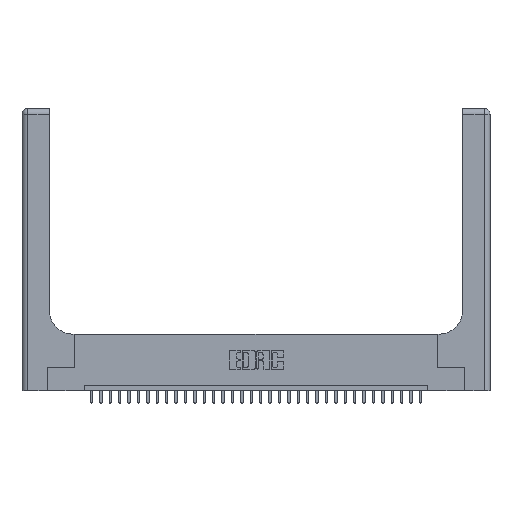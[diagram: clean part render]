
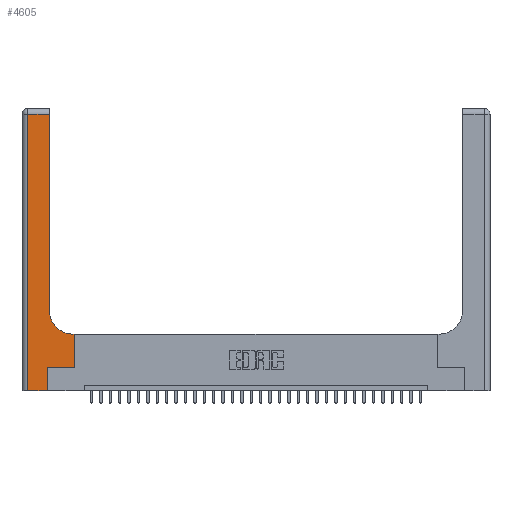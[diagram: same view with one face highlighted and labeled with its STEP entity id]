
A CAD part, top view. The second image highlights one B-rep face of the part: STEP entity #4605.
In plain terms, the highlighted planar face has unit normal (0, 0, 1).
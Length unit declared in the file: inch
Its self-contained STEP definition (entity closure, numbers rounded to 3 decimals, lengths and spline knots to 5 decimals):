
#498 = VERTEX_POINT ( 'NONE', #14320 ) ;
#702 = EDGE_CURVE ( 'NONE', #2515, #7853, #27507, .T. ) ;
#798 = DIRECTION ( 'NONE',  ( 1., 0., 0. ) ) ;
#1124 = CARTESIAN_POINT ( 'NONE',  ( 0.269, 0., 0.37 ) ) ;
#1391 = LINE ( 'NONE', #16752, #14208 ) ;
#1952 = VECTOR ( 'NONE', #13295, 39.37008 ) ;
#2410 = CARTESIAN_POINT ( 'NONE',  ( 0.5585, 0.25, 0.37 ) ) ;
#2515 = VERTEX_POINT ( 'NONE', #7560 ) ;
#3323 = CIRCLE ( 'NONE', #4582, 0.25 ) ;
#4096 = FACE_OUTER_BOUND ( 'NONE', #16424, .T. ) ;
#4129 = AXIS2_PLACEMENT_3D ( 'NONE', #18229, #7940, #10505 ) ;
#4148 = CARTESIAN_POINT ( 'NONE',  ( 0.269, 0.25, 0.37 ) ) ;
#4215 = LINE ( 'NONE', #9940, #5830 ) ;
#4252 = ORIENTED_EDGE ( 'NONE', *, *, #15939, .T. ) ;
#4377 = CARTESIAN_POINT ( 'NONE',  ( 0.269, 0., 0.37 ) ) ;
#4383 = CARTESIAN_POINT ( 'NONE',  ( 0.2915, 0.85, 0.37 ) ) ;
#4582 = AXIS2_PLACEMENT_3D ( 'NONE', #7587, #17984, #17672 ) ;
#4605 = ADVANCED_FACE ( 'NONE', ( #4096 ), #30809, .F. ) ;
#4661 = CARTESIAN_POINT ( 'NONE',  ( 0.5585, 0.25, 0.37 ) ) ;
#5014 = DIRECTION ( 'NONE',  ( 0., 1., 0. ) ) ;
#5274 = ORIENTED_EDGE ( 'NONE', *, *, #17654, .T. ) ;
#5356 = VECTOR ( 'NONE', #23576, 39.37008 ) ;
#5830 = VECTOR ( 'NONE', #15091, 39.37008 ) ;
#7560 = CARTESIAN_POINT ( 'NONE',  ( 0.06, 0., 0.37 ) ) ;
#7587 = CARTESIAN_POINT ( 'NONE',  ( 0.5415, 0.85, 0.37 ) ) ;
#7853 = VERTEX_POINT ( 'NONE', #1124 ) ;
#7940 = DIRECTION ( 'NONE',  ( 0., 0., -1. ) ) ;
#8458 = EDGE_CURVE ( 'NONE', #22135, #18496, #20179, .T. ) ;
#9336 = EDGE_CURVE ( 'NONE', #12132, #498, #11355, .T. ) ;
#9940 = CARTESIAN_POINT ( 'NONE',  ( 0.2915, 0.6, 0.37 ) ) ;
#10505 = DIRECTION ( 'NONE',  ( -1., 0., 0. ) ) ;
#10532 = VERTEX_POINT ( 'NONE', #10680 ) ;
#10680 = CARTESIAN_POINT ( 'NONE',  ( 0.06, 2.94, 0.37 ) ) ;
#11167 = EDGE_CURVE ( 'NONE', #7853, #28738, #30779, .T. ) ;
#11355 = LINE ( 'NONE', #13648, #5356 ) ;
#11925 = DIRECTION ( 'NONE',  ( 0., -1., 0. ) ) ;
#12132 = VERTEX_POINT ( 'NONE', #4383 ) ;
#12150 = DIRECTION ( 'NONE',  ( -1., 0., 0. ) ) ;
#12954 = CARTESIAN_POINT ( 'NONE',  ( 0., 0., 0.37 ) ) ;
#13295 = DIRECTION ( 'NONE',  ( 1., 0., 0. ) ) ;
#13648 = CARTESIAN_POINT ( 'NONE',  ( 0.2915, 3., 0.37 ) ) ;
#14208 = VECTOR ( 'NONE', #11925, 39.37008 ) ;
#14320 = CARTESIAN_POINT ( 'NONE',  ( 0.2915, 2.94, 0.37 ) ) ;
#15091 = DIRECTION ( 'NONE',  ( -1., 0., 0. ) ) ;
#15939 = EDGE_CURVE ( 'NONE', #31539, #12132, #3323, .T. ) ;
#16143 = CARTESIAN_POINT ( 'NONE',  ( 0.269, 0.25, 0.37 ) ) ;
#16424 = EDGE_LOOP ( 'NONE', ( #26252, #26799, #16755, #18764, #23884, #5274, #21580, #23521, #4252 ) ) ;
#16752 = CARTESIAN_POINT ( 'NONE',  ( 0.06, 3., 0.37 ) ) ;
#16755 = ORIENTED_EDGE ( 'NONE', *, *, #31317, .T. ) ;
#17266 = DIRECTION ( 'NONE',  ( 0., 1., 0. ) ) ;
#17654 = EDGE_CURVE ( 'NONE', #28738, #22135, #20352, .T. ) ;
#17672 = DIRECTION ( 'NONE',  ( 1., 0., 0. ) ) ;
#17984 = DIRECTION ( 'NONE',  ( 0., 0., -1. ) ) ;
#18052 = CARTESIAN_POINT ( 'NONE',  ( 0.5585, 0.6, 0.37 ) ) ;
#18229 = CARTESIAN_POINT ( 'NONE',  ( 0., 3., 0.37 ) ) ;
#18496 = VERTEX_POINT ( 'NONE', #18052 ) ;
#18764 = ORIENTED_EDGE ( 'NONE', *, *, #702, .T. ) ;
#20179 = LINE ( 'NONE', #2410, #32966 ) ;
#20352 = LINE ( 'NONE', #16143, #32337 ) ;
#21580 = ORIENTED_EDGE ( 'NONE', *, *, #8458, .T. ) ;
#22047 = VECTOR ( 'NONE', #17266, 39.37008 ) ;
#22135 = VERTEX_POINT ( 'NONE', #4661 ) ;
#22917 = EDGE_CURVE ( 'NONE', #498, #10532, #30560, .T. ) ;
#23521 = ORIENTED_EDGE ( 'NONE', *, *, #30892, .T. ) ;
#23576 = DIRECTION ( 'NONE',  ( 0., 1., 0. ) ) ;
#23884 = ORIENTED_EDGE ( 'NONE', *, *, #11167, .T. ) ;
#26252 = ORIENTED_EDGE ( 'NONE', *, *, #9336, .T. ) ;
#26799 = ORIENTED_EDGE ( 'NONE', *, *, #22917, .T. ) ;
#27507 = LINE ( 'NONE', #12954, #1952 ) ;
#28738 = VERTEX_POINT ( 'NONE', #4148 ) ;
#30560 = LINE ( 'NONE', #33130, #32161 ) ;
#30779 = LINE ( 'NONE', #4377, #22047 ) ;
#30809 = PLANE ( 'NONE',  #4129 ) ;
#30855 = CARTESIAN_POINT ( 'NONE',  ( 0.5415, 0.6, 0.37 ) ) ;
#30892 = EDGE_CURVE ( 'NONE', #18496, #31539, #4215, .T. ) ;
#31317 = EDGE_CURVE ( 'NONE', #10532, #2515, #1391, .T. ) ;
#31539 = VERTEX_POINT ( 'NONE', #30855 ) ;
#32161 = VECTOR ( 'NONE', #12150, 39.37008 ) ;
#32337 = VECTOR ( 'NONE', #798, 39.37008 ) ;
#32966 = VECTOR ( 'NONE', #5014, 39.37008 ) ;
#33130 = CARTESIAN_POINT ( 'NONE',  ( 0., 2.94, 0.37 ) ) ;
